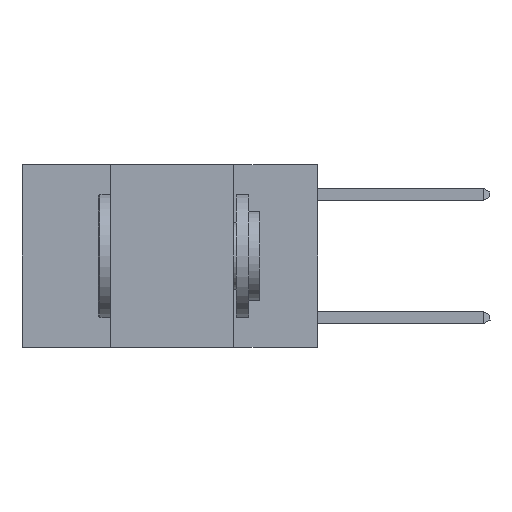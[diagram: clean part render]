
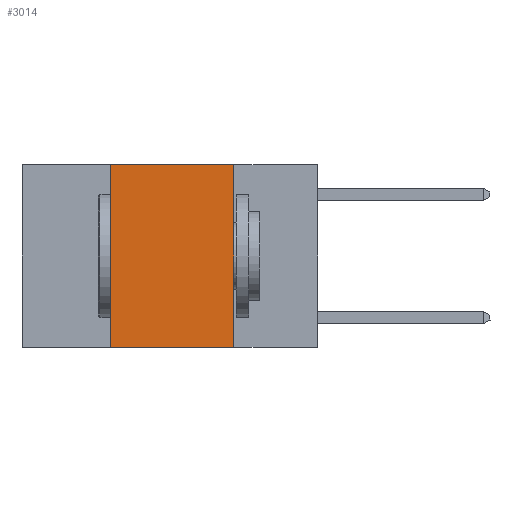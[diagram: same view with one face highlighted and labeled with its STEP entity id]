
A CAD part, left-side view. The second image highlights one B-rep face of the part: STEP entity #3014.
In plain terms, the highlighted planar face has unit normal (-1, 0, 0).
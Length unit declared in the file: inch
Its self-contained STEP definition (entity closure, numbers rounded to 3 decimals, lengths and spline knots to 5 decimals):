
#1840 = DIRECTION ( 'NONE',  ( 0., 0., -1. ) ) ;
#2224 = PLANE ( 'NONE',  #5706 ) ;
#2334 = CARTESIAN_POINT ( 'NONE',  ( 0., 0.17, -0.37 ) ) ;
#2997 = EDGE_CURVE ( 'NONE', #4611, #8448, #3060, .T. ) ;
#3014 = ADVANCED_FACE ( 'NONE', ( #8644 ), #2224, .F. ) ;
#3060 = LINE ( 'NONE', #12563, #14015 ) ;
#4367 = EDGE_CURVE ( 'NONE', #8448, #4523, #5320, .T. ) ;
#4523 = VERTEX_POINT ( 'NONE', #14306 ) ;
#4611 = VERTEX_POINT ( 'NONE', #20317 ) ;
#4893 = ORIENTED_EDGE ( 'NONE', *, *, #4957, .T. ) ;
#4957 = EDGE_CURVE ( 'NONE', #4611, #16421, #18804, .T. ) ;
#5320 = LINE ( 'NONE', #22416, #14910 ) ;
#5329 = LINE ( 'NONE', #5964, #25508 ) ;
#5706 = AXIS2_PLACEMENT_3D ( 'NONE', #16522, #10616, #24081 ) ;
#5964 = CARTESIAN_POINT ( 'NONE',  ( 0., 0.17, 0. ) ) ;
#7841 = ORIENTED_EDGE ( 'NONE', *, *, #12829, .F. ) ;
#8448 = VERTEX_POINT ( 'NONE', #8709 ) ;
#8644 = FACE_OUTER_BOUND ( 'NONE', #23533, .T. ) ;
#8709 = CARTESIAN_POINT ( 'NONE',  ( 0., 0.42, 0. ) ) ;
#9444 = CARTESIAN_POINT ( 'NONE',  ( 0., 0.6, -0.37 ) ) ;
#10616 = DIRECTION ( 'NONE',  ( 1., 0., 0. ) ) ;
#12563 = CARTESIAN_POINT ( 'NONE',  ( 0., 0.42, 0. ) ) ;
#12829 = EDGE_CURVE ( 'NONE', #4523, #16421, #5329, .T. ) ;
#13629 = VECTOR ( 'NONE', #15468, 39.37008 ) ;
#14015 = VECTOR ( 'NONE', #14553, 39.37008 ) ;
#14306 = CARTESIAN_POINT ( 'NONE',  ( 0., 0.17, 0. ) ) ;
#14553 = DIRECTION ( 'NONE',  ( 0., 0., 1. ) ) ;
#14910 = VECTOR ( 'NONE', #20493, 39.37008 ) ;
#15468 = DIRECTION ( 'NONE',  ( 0., -1., 0. ) ) ;
#16421 = VERTEX_POINT ( 'NONE', #2334 ) ;
#16522 = CARTESIAN_POINT ( 'NONE',  ( 0., 0.6, 0. ) ) ;
#18804 = LINE ( 'NONE', #9444, #13629 ) ;
#19593 = ORIENTED_EDGE ( 'NONE', *, *, #2997, .F. ) ;
#20317 = CARTESIAN_POINT ( 'NONE',  ( 0., 0.42, -0.37 ) ) ;
#20493 = DIRECTION ( 'NONE',  ( 0., -1., 0. ) ) ;
#22416 = CARTESIAN_POINT ( 'NONE',  ( 0., 0.6, 0. ) ) ;
#23394 = ORIENTED_EDGE ( 'NONE', *, *, #4367, .F. ) ;
#23533 = EDGE_LOOP ( 'NONE', ( #7841, #23394, #19593, #4893 ) ) ;
#24081 = DIRECTION ( 'NONE',  ( 0., 0., -1. ) ) ;
#25508 = VECTOR ( 'NONE', #1840, 39.37008 ) ;
